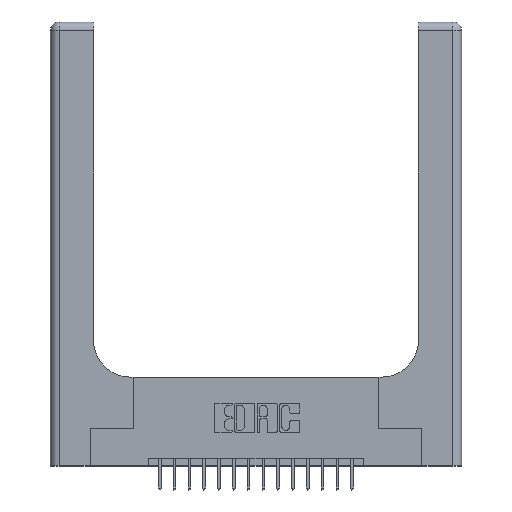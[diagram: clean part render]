
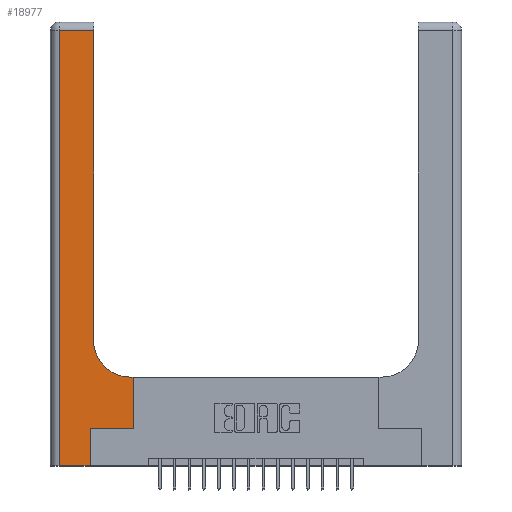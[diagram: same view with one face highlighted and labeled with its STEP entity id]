
A CAD part, top view. The second image highlights one B-rep face of the part: STEP entity #18977.
In plain terms, the highlighted planar face has unit normal (0, 0, 1).
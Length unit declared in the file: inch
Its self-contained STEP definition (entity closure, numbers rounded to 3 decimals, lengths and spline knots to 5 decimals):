
#120 = DIRECTION ( 'NONE',  ( 0., 0., -1. ) ) ;
#143 = EDGE_CURVE ( 'NONE', #7156, #15854, #7258, .T. ) ;
#206 = VECTOR ( 'NONE', #16864, 39.37008 ) ;
#369 = VERTEX_POINT ( 'NONE', #6617 ) ;
#551 = CARTESIAN_POINT ( 'NONE',  ( 0.5585, 0.25, 0.37 ) ) ;
#699 = EDGE_CURVE ( 'NONE', #3531, #5452, #7514, .T. ) ;
#1326 = CARTESIAN_POINT ( 'NONE',  ( 0., 2.94, 0.37 ) ) ;
#1554 = EDGE_CURVE ( 'NONE', #7626, #3531, #19627, .T. ) ;
#1820 = VERTEX_POINT ( 'NONE', #15046 ) ;
#2082 = VECTOR ( 'NONE', #10609, 39.37008 ) ;
#2791 = FACE_OUTER_BOUND ( 'NONE', #16290, .T. ) ;
#3263 = DIRECTION ( 'NONE',  ( -1., 0., 0. ) ) ;
#3353 = VECTOR ( 'NONE', #14811, 39.37008 ) ;
#3531 = VERTEX_POINT ( 'NONE', #18582 ) ;
#3603 = CARTESIAN_POINT ( 'NONE',  ( 0.06, 3., 0.37 ) ) ;
#3636 = EDGE_CURVE ( 'NONE', #369, #1820, #12211, .T. ) ;
#4000 = EDGE_CURVE ( 'NONE', #15854, #5533, #13399, .T. ) ;
#4087 = VECTOR ( 'NONE', #4848, 39.37008 ) ;
#4728 = CARTESIAN_POINT ( 'NONE',  ( 0.5415, 0.85, 0.37 ) ) ;
#4848 = DIRECTION ( 'NONE',  ( 0., 1., 0. ) ) ;
#5054 = LINE ( 'NONE', #17103, #16716 ) ;
#5452 = VERTEX_POINT ( 'NONE', #551 ) ;
#5533 = VERTEX_POINT ( 'NONE', #13180 ) ;
#5615 = CARTESIAN_POINT ( 'NONE',  ( 0., 0., 0.37 ) ) ;
#6222 = PLANE ( 'NONE',  #17786 ) ;
#6247 = EDGE_CURVE ( 'NONE', #5452, #10646, #6533, .T. ) ;
#6352 = ORIENTED_EDGE ( 'NONE', *, *, #11594, .T. ) ;
#6533 = LINE ( 'NONE', #11547, #3353 ) ;
#6571 = ORIENTED_EDGE ( 'NONE', *, *, #15474, .T. ) ;
#6617 = CARTESIAN_POINT ( 'NONE',  ( 0.06, 2.94, 0.37 ) ) ;
#6912 = CARTESIAN_POINT ( 'NONE',  ( 0.269, 0., 0.37 ) ) ;
#7156 = VERTEX_POINT ( 'NONE', #10300 ) ;
#7258 = CIRCLE ( 'NONE', #9875, 0.25 ) ;
#7514 = LINE ( 'NONE', #18007, #10589 ) ;
#7626 = VERTEX_POINT ( 'NONE', #6912 ) ;
#7679 = VECTOR ( 'NONE', #13361, 39.37008 ) ;
#7743 = ORIENTED_EDGE ( 'NONE', *, *, #11501, .T. ) ;
#7811 = DIRECTION ( 'NONE',  ( -1., 0., 0. ) ) ;
#7842 = DIRECTION ( 'NONE',  ( 1., 0., 0. ) ) ;
#9875 = AXIS2_PLACEMENT_3D ( 'NONE', #4728, #18162, #7842 ) ;
#10271 = DIRECTION ( 'NONE',  ( 1., 0., 0. ) ) ;
#10300 = CARTESIAN_POINT ( 'NONE',  ( 0.5415, 0.6, 0.37 ) ) ;
#10384 = ORIENTED_EDGE ( 'NONE', *, *, #3636, .T. ) ;
#10589 = VECTOR ( 'NONE', #10271, 39.37008 ) ;
#10609 = DIRECTION ( 'NONE',  ( 0., 1., 0. ) ) ;
#10646 = VERTEX_POINT ( 'NONE', #14773 ) ;
#11268 = LINE ( 'NONE', #1326, #206 ) ;
#11501 = EDGE_CURVE ( 'NONE', #1820, #7626, #17851, .T. ) ;
#11547 = CARTESIAN_POINT ( 'NONE',  ( 0.5585, 0.25, 0.37 ) ) ;
#11594 = EDGE_CURVE ( 'NONE', #5533, #369, #11268, .T. ) ;
#12211 = LINE ( 'NONE', #3603, #18312 ) ;
#12555 = CARTESIAN_POINT ( 'NONE',  ( 0., 3., 0.37 ) ) ;
#13180 = CARTESIAN_POINT ( 'NONE',  ( 0.2915, 2.94, 0.37 ) ) ;
#13361 = DIRECTION ( 'NONE',  ( 1., 0., 0. ) ) ;
#13399 = LINE ( 'NONE', #13949, #2082 ) ;
#13949 = CARTESIAN_POINT ( 'NONE',  ( 0.2915, 3., 0.37 ) ) ;
#14188 = ORIENTED_EDGE ( 'NONE', *, *, #4000, .T. ) ;
#14409 = DIRECTION ( 'NONE',  ( 0., -1., 0. ) ) ;
#14773 = CARTESIAN_POINT ( 'NONE',  ( 0.5585, 0.6, 0.37 ) ) ;
#14811 = DIRECTION ( 'NONE',  ( 0., 1., 0. ) ) ;
#14837 = ORIENTED_EDGE ( 'NONE', *, *, #699, .T. ) ;
#15046 = CARTESIAN_POINT ( 'NONE',  ( 0.06, 0., 0.37 ) ) ;
#15402 = CARTESIAN_POINT ( 'NONE',  ( 0.269, 0., 0.37 ) ) ;
#15474 = EDGE_CURVE ( 'NONE', #10646, #7156, #5054, .T. ) ;
#15854 = VERTEX_POINT ( 'NONE', #19355 ) ;
#16290 = EDGE_LOOP ( 'NONE', ( #14188, #6352, #10384, #7743, #16462, #14837, #19548, #6571, #19317 ) ) ;
#16462 = ORIENTED_EDGE ( 'NONE', *, *, #1554, .T. ) ;
#16716 = VECTOR ( 'NONE', #7811, 39.37008 ) ;
#16864 = DIRECTION ( 'NONE',  ( -1., 0., 0. ) ) ;
#17103 = CARTESIAN_POINT ( 'NONE',  ( 0.2915, 0.6, 0.37 ) ) ;
#17786 = AXIS2_PLACEMENT_3D ( 'NONE', #12555, #120, #3263 ) ;
#17851 = LINE ( 'NONE', #5615, #7679 ) ;
#18007 = CARTESIAN_POINT ( 'NONE',  ( 0.269, 0.25, 0.37 ) ) ;
#18162 = DIRECTION ( 'NONE',  ( 0., 0., -1. ) ) ;
#18312 = VECTOR ( 'NONE', #14409, 39.37008 ) ;
#18582 = CARTESIAN_POINT ( 'NONE',  ( 0.269, 0.25, 0.37 ) ) ;
#18977 = ADVANCED_FACE ( 'NONE', ( #2791 ), #6222, .F. ) ;
#19317 = ORIENTED_EDGE ( 'NONE', *, *, #143, .T. ) ;
#19355 = CARTESIAN_POINT ( 'NONE',  ( 0.2915, 0.85, 0.37 ) ) ;
#19548 = ORIENTED_EDGE ( 'NONE', *, *, #6247, .T. ) ;
#19627 = LINE ( 'NONE', #15402, #4087 ) ;
